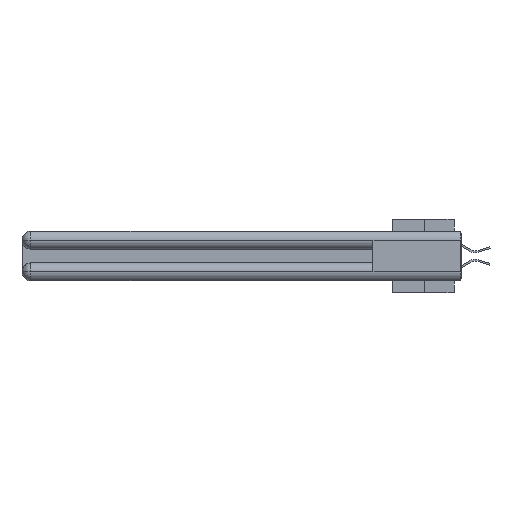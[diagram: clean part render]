
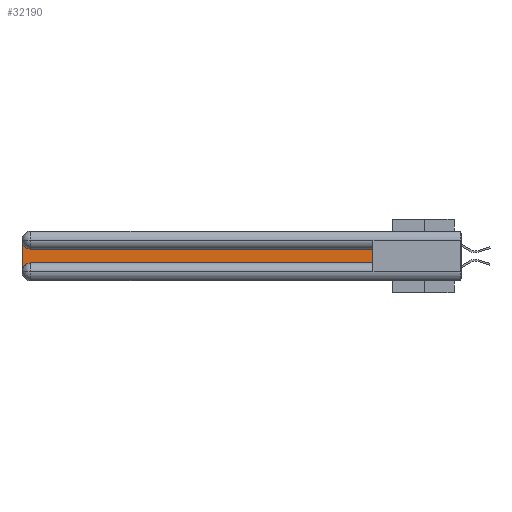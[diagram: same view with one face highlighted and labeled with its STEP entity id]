
A CAD part, left-side view. The second image highlights one B-rep face of the part: STEP entity #32190.
In plain terms, the highlighted planar face has unit normal (-1, 0, 0).
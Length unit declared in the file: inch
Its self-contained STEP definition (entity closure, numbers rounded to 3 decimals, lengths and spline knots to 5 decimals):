
#1259 = CARTESIAN_POINT ( 'NONE',  ( 0.075, 3., -0.2175 ) ) ;
#2825 = EDGE_CURVE ( 'NONE', #26390, #3365, #20933, .T. ) ;
#3365 = VERTEX_POINT ( 'NONE', #18809 ) ;
#3419 = CARTESIAN_POINT ( 'NONE',  ( 0.075, 2.94, -0.2775 ) ) ;
#3543 = DIRECTION ( 'NONE',  ( 0., 0., -1. ) ) ;
#3903 = VECTOR ( 'NONE', #26566, 39.37008 ) ;
#4386 = PLANE ( 'NONE',  #24062 ) ;
#5147 = EDGE_CURVE ( 'NONE', #32814, #23989, #15918, .T. ) ;
#5390 = ORIENTED_EDGE ( 'NONE', *, *, #21262, .T. ) ;
#6033 = LINE ( 'NONE', #26445, #20919 ) ;
#6383 = AXIS2_PLACEMENT_3D ( 'NONE', #9849, #20915, #18344 ) ;
#6596 = DIRECTION ( 'NONE',  ( 0., 0., -1. ) ) ;
#7537 = CARTESIAN_POINT ( 'NONE',  ( 0.075, 0.6, -0.1225 ) ) ;
#7780 = EDGE_CURVE ( 'NONE', #23989, #15411, #16356, .T. ) ;
#9067 = FACE_OUTER_BOUND ( 'NONE', #18187, .T. ) ;
#9849 = CARTESIAN_POINT ( 'NONE',  ( 0.075, 2.94, -0.0625 ) ) ;
#10293 = CARTESIAN_POINT ( 'NONE',  ( 0.075, 3., -0.0625 ) ) ;
#10568 = ORIENTED_EDGE ( 'NONE', *, *, #10977, .T. ) ;
#10977 = EDGE_CURVE ( 'NONE', #11131, #32814, #6033, .T. ) ;
#11131 = VERTEX_POINT ( 'NONE', #7537 ) ;
#15411 = VERTEX_POINT ( 'NONE', #30812 ) ;
#15918 = CIRCLE ( 'NONE', #6383, 0.06 ) ;
#16116 = DIRECTION ( 'NONE',  ( 0., 0., 1. ) ) ;
#16356 = LINE ( 'NONE', #1259, #17658 ) ;
#16539 = CARTESIAN_POINT ( 'NONE',  ( 0.075, 2.94, -0.2175 ) ) ;
#17658 = VECTOR ( 'NONE', #6596, 39.37008 ) ;
#18187 = EDGE_LOOP ( 'NONE', ( #10568, #22198, #21885, #28119, #19169, #5390 ) ) ;
#18344 = DIRECTION ( 'NONE',  ( 0., 0., -1. ) ) ;
#18809 = CARTESIAN_POINT ( 'NONE',  ( 0.075, 0.6, -0.2175 ) ) ;
#19169 = ORIENTED_EDGE ( 'NONE', *, *, #2825, .T. ) ;
#20716 = CARTESIAN_POINT ( 'NONE',  ( 0.075, 2.94, -0.1225 ) ) ;
#20915 = DIRECTION ( 'NONE',  ( 1., 0., 0. ) ) ;
#20919 = VECTOR ( 'NONE', #26824, 39.37008 ) ;
#20933 = LINE ( 'NONE', #29151, #3903 ) ;
#21262 = EDGE_CURVE ( 'NONE', #3365, #11131, #29112, .T. ) ;
#21885 = ORIENTED_EDGE ( 'NONE', *, *, #7780, .T. ) ;
#22198 = ORIENTED_EDGE ( 'NONE', *, *, #5147, .T. ) ;
#23989 = VERTEX_POINT ( 'NONE', #10293 ) ;
#24062 = AXIS2_PLACEMENT_3D ( 'NONE', #29614, #32199, #35274 ) ;
#26291 = DIRECTION ( 'NONE',  ( 1., 0., 0. ) ) ;
#26390 = VERTEX_POINT ( 'NONE', #16539 ) ;
#26445 = CARTESIAN_POINT ( 'NONE',  ( 0.075, 0.6, -0.1225 ) ) ;
#26566 = DIRECTION ( 'NONE',  ( 0., -1., 0. ) ) ;
#26824 = DIRECTION ( 'NONE',  ( 0., 1., 0. ) ) ;
#27132 = CIRCLE ( 'NONE', #34177, 0.06 ) ;
#28119 = ORIENTED_EDGE ( 'NONE', *, *, #31355, .T. ) ;
#29112 = LINE ( 'NONE', #35668, #29528 ) ;
#29151 = CARTESIAN_POINT ( 'NONE',  ( 0.075, 0.6, -0.2175 ) ) ;
#29528 = VECTOR ( 'NONE', #16116, 39.37008 ) ;
#29614 = CARTESIAN_POINT ( 'NONE',  ( 0.075, 3., -0.1225 ) ) ;
#30812 = CARTESIAN_POINT ( 'NONE',  ( 0.075, 3., -0.2775 ) ) ;
#31355 = EDGE_CURVE ( 'NONE', #15411, #26390, #27132, .T. ) ;
#32190 = ADVANCED_FACE ( 'NONE', ( #9067 ), #4386, .F. ) ;
#32199 = DIRECTION ( 'NONE',  ( 1., 0., 0. ) ) ;
#32814 = VERTEX_POINT ( 'NONE', #20716 ) ;
#34177 = AXIS2_PLACEMENT_3D ( 'NONE', #3419, #26291, #3543 ) ;
#35274 = DIRECTION ( 'NONE',  ( 0., 0., -1. ) ) ;
#35668 = CARTESIAN_POINT ( 'NONE',  ( 0.075, 0.6, -0.2175 ) ) ;
